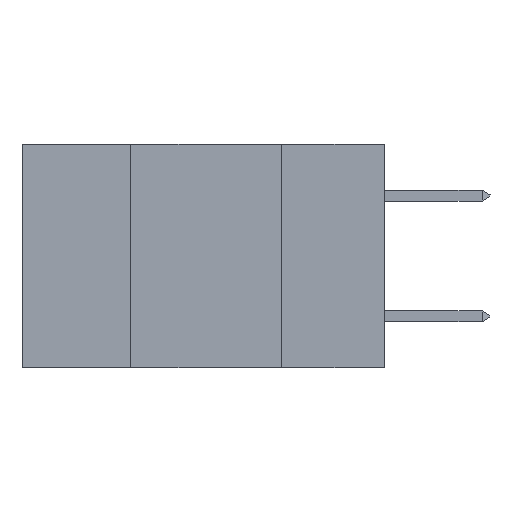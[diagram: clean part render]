
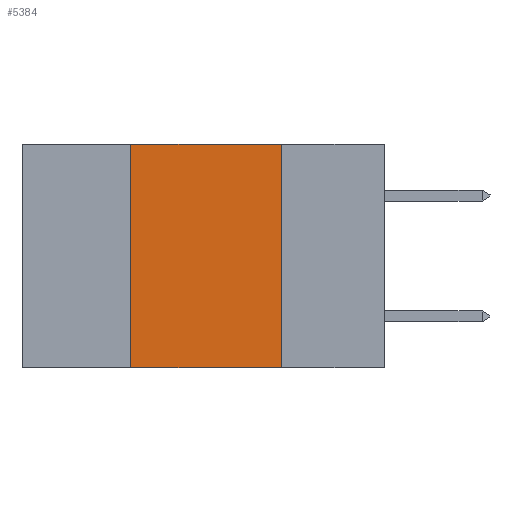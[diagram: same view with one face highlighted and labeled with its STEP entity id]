
A CAD part, left-side view. The second image highlights one B-rep face of the part: STEP entity #5384.
In plain terms, the highlighted planar face has unit normal (-1, 0, 0).
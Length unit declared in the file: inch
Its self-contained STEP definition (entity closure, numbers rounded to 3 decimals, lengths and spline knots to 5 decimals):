
#450 = EDGE_CURVE ( 'NONE', #20873, #2157, #13630, .T. ) ;
#1909 = CARTESIAN_POINT ( 'NONE',  ( 0., 0.6, -0.37 ) ) ;
#2104 = AXIS2_PLACEMENT_3D ( 'NONE', #5070, #17883, #40330 ) ;
#2125 = ORIENTED_EDGE ( 'NONE', *, *, #33348, .T. ) ;
#2157 = VERTEX_POINT ( 'NONE', #25999 ) ;
#3664 = CARTESIAN_POINT ( 'NONE',  ( 0., 0.6, 0. ) ) ;
#3734 = VERTEX_POINT ( 'NONE', #33161 ) ;
#4680 = VECTOR ( 'NONE', #28667, 39.37008 ) ;
#5070 = CARTESIAN_POINT ( 'NONE',  ( 0., 0.6, 0. ) ) ;
#5384 = ADVANCED_FACE ( 'NONE', ( #8631 ), #21032, .F. ) ;
#8346 = ORIENTED_EDGE ( 'NONE', *, *, #450, .F. ) ;
#8631 = FACE_OUTER_BOUND ( 'NONE', #15768, .T. ) ;
#8780 = DIRECTION ( 'NONE',  ( 0., 0., 1. ) ) ;
#9334 = VECTOR ( 'NONE', #24773, 39.37008 ) ;
#12681 = LINE ( 'NONE', #3664, #4680 ) ;
#13630 = LINE ( 'NONE', #20358, #30555 ) ;
#13825 = CARTESIAN_POINT ( 'NONE',  ( 0., 0.17, 0. ) ) ;
#14765 = VERTEX_POINT ( 'NONE', #40128 ) ;
#15768 = EDGE_LOOP ( 'NONE', ( #8346, #25267, #30776, #2125 ) ) ;
#17883 = DIRECTION ( 'NONE',  ( 1., 0., 0. ) ) ;
#20358 = CARTESIAN_POINT ( 'NONE',  ( 0., 0.17, 0. ) ) ;
#20803 = LINE ( 'NONE', #1909, #9334 ) ;
#20873 = VERTEX_POINT ( 'NONE', #13825 ) ;
#20979 = LINE ( 'NONE', #40275, #34794 ) ;
#21032 = PLANE ( 'NONE',  #2104 ) ;
#24773 = DIRECTION ( 'NONE',  ( 0., -1., 0. ) ) ;
#25267 = ORIENTED_EDGE ( 'NONE', *, *, #41407, .F. ) ;
#25999 = CARTESIAN_POINT ( 'NONE',  ( 0., 0.17, -0.37 ) ) ;
#28667 = DIRECTION ( 'NONE',  ( 0., -1., 0. ) ) ;
#29800 = DIRECTION ( 'NONE',  ( 0., 0., -1. ) ) ;
#30555 = VECTOR ( 'NONE', #29800, 39.37008 ) ;
#30776 = ORIENTED_EDGE ( 'NONE', *, *, #32315, .F. ) ;
#32315 = EDGE_CURVE ( 'NONE', #14765, #3734, #20979, .T. ) ;
#33161 = CARTESIAN_POINT ( 'NONE',  ( 0., 0.42, 0. ) ) ;
#33348 = EDGE_CURVE ( 'NONE', #14765, #2157, #20803, .T. ) ;
#34794 = VECTOR ( 'NONE', #8780, 39.37008 ) ;
#40128 = CARTESIAN_POINT ( 'NONE',  ( 0., 0.42, -0.37 ) ) ;
#40275 = CARTESIAN_POINT ( 'NONE',  ( 0., 0.42, 0. ) ) ;
#40330 = DIRECTION ( 'NONE',  ( 0., 0., -1. ) ) ;
#41407 = EDGE_CURVE ( 'NONE', #3734, #20873, #12681, .T. ) ;
